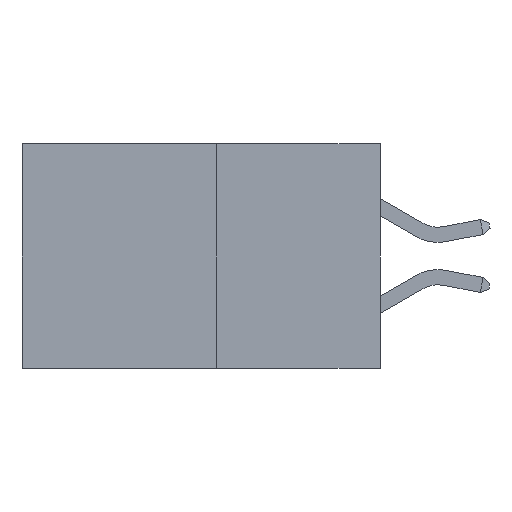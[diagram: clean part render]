
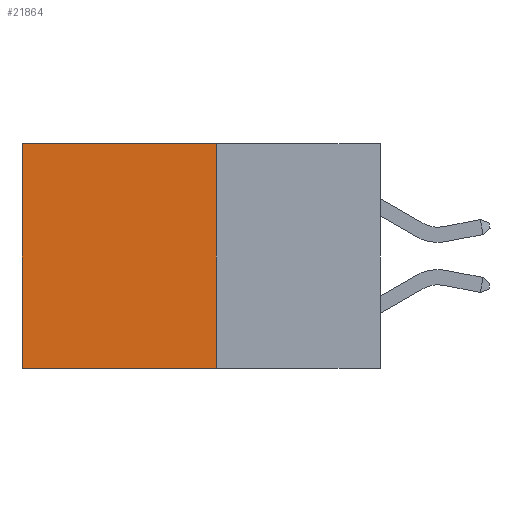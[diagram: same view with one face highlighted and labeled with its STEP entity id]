
A CAD part, left-side view. The second image highlights one B-rep face of the part: STEP entity #21864.
In plain terms, the highlighted planar face has unit normal (-1, 0, 0).
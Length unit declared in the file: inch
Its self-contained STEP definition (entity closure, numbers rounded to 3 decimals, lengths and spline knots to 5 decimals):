
#103 = AXIS2_PLACEMENT_3D ( 'NONE', #3257, #15832, #5086 ) ;
#1191 = VECTOR ( 'NONE', #17775, 39.37008 ) ;
#1221 = LINE ( 'NONE', #16323, #5485 ) ;
#1441 = PLANE ( 'NONE',  #103 ) ;
#1715 = VECTOR ( 'NONE', #3672, 39.37008 ) ;
#2291 = LINE ( 'NONE', #22747, #1715 ) ;
#3257 = CARTESIAN_POINT ( 'NONE',  ( 0.277, 0.27, -0.37 ) ) ;
#3345 = EDGE_CURVE ( 'NONE', #22340, #3994, #2291, .T. ) ;
#3408 = CARTESIAN_POINT ( 'NONE',  ( 0.277, 0.27, -0.37 ) ) ;
#3672 = DIRECTION ( 'NONE',  ( 0., 1., 0. ) ) ;
#3994 = VERTEX_POINT ( 'NONE', #18376 ) ;
#4529 = VERTEX_POINT ( 'NONE', #5291 ) ;
#4694 = CARTESIAN_POINT ( 'NONE',  ( 0.277, 0.27, 0. ) ) ;
#5086 = DIRECTION ( 'NONE',  ( 0., 0., -1. ) ) ;
#5291 = CARTESIAN_POINT ( 'NONE',  ( 0.277, 0.27, 0. ) ) ;
#5485 = VECTOR ( 'NONE', #9235, 39.37008 ) ;
#5962 = CARTESIAN_POINT ( 'NONE',  ( 0.277, 0.59, 0. ) ) ;
#7132 = ORIENTED_EDGE ( 'NONE', *, *, #11691, .T. ) ;
#8308 = EDGE_LOOP ( 'NONE', ( #7132, #11942, #17760, #13848 ) ) ;
#8604 = VECTOR ( 'NONE', #22469, 39.37008 ) ;
#9235 = DIRECTION ( 'NONE',  ( 0., 0., -1. ) ) ;
#11691 = EDGE_CURVE ( 'NONE', #12504, #3994, #1221, .T. ) ;
#11942 = ORIENTED_EDGE ( 'NONE', *, *, #3345, .F. ) ;
#12504 = VERTEX_POINT ( 'NONE', #5962 ) ;
#13503 = CARTESIAN_POINT ( 'NONE',  ( 0.277, 0.27, -0.37 ) ) ;
#13848 = ORIENTED_EDGE ( 'NONE', *, *, #19256, .T. ) ;
#15568 = LINE ( 'NONE', #3408, #1191 ) ;
#15832 = DIRECTION ( 'NONE',  ( 1., 0., 0. ) ) ;
#16323 = CARTESIAN_POINT ( 'NONE',  ( 0.277, 0.59, -0.37 ) ) ;
#17760 = ORIENTED_EDGE ( 'NONE', *, *, #20008, .F. ) ;
#17775 = DIRECTION ( 'NONE',  ( 0., 0., -1. ) ) ;
#18376 = CARTESIAN_POINT ( 'NONE',  ( 0.277, 0.59, -0.37 ) ) ;
#18659 = LINE ( 'NONE', #4694, #8604 ) ;
#19256 = EDGE_CURVE ( 'NONE', #4529, #12504, #18659, .T. ) ;
#20008 = EDGE_CURVE ( 'NONE', #4529, #22340, #15568, .T. ) ;
#21342 = FACE_OUTER_BOUND ( 'NONE', #8308, .T. ) ;
#21864 = ADVANCED_FACE ( 'NONE', ( #21342 ), #1441, .F. ) ;
#22340 = VERTEX_POINT ( 'NONE', #13503 ) ;
#22469 = DIRECTION ( 'NONE',  ( 0., 1., 0. ) ) ;
#22747 = CARTESIAN_POINT ( 'NONE',  ( 0.277, 0.27, -0.37 ) ) ;
